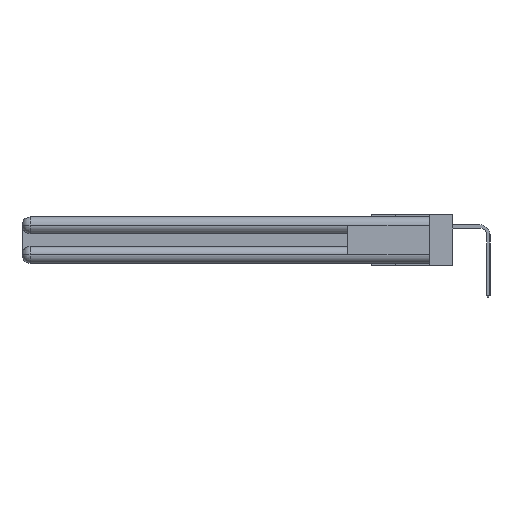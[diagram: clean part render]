
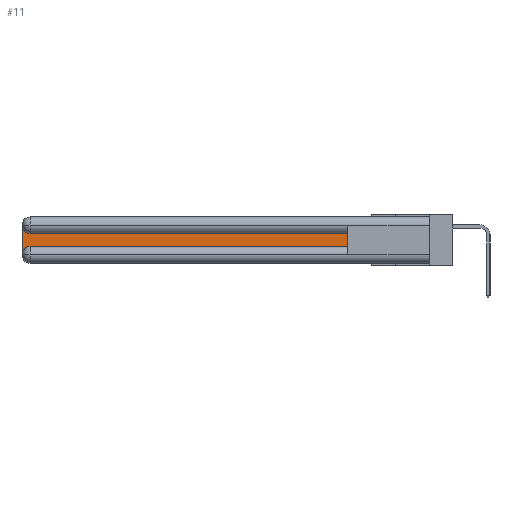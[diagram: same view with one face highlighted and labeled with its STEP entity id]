
A CAD part, left-side view. The second image highlights one B-rep face of the part: STEP entity #11.
In plain terms, the highlighted planar face has unit normal (-1, 0, 0).
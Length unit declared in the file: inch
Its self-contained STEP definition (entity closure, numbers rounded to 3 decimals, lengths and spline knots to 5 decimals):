
#11 = ADVANCED_FACE ( 'NONE', ( #14824 ), #11236, .F. ) ;
#300 = DIRECTION ( 'NONE',  ( 1., 0., 0. ) ) ;
#1218 = DIRECTION ( 'NONE',  ( 1., 0., 0. ) ) ;
#1413 = VECTOR ( 'NONE', #3576, 39.37008 ) ;
#2156 = VECTOR ( 'NONE', #27967, 39.37008 ) ;
#2687 = VECTOR ( 'NONE', #27458, 39.37008 ) ;
#2861 = VERTEX_POINT ( 'NONE', #9665 ) ;
#3286 = ORIENTED_EDGE ( 'NONE', *, *, #26084, .T. ) ;
#3576 = DIRECTION ( 'NONE',  ( 0., 0., 1. ) ) ;
#4928 = LINE ( 'NONE', #28061, #2156 ) ;
#5593 = CARTESIAN_POINT ( 'NONE',  ( 0.075, 0.6, -0.2175 ) ) ;
#7608 = VERTEX_POINT ( 'NONE', #24763 ) ;
#7755 = ORIENTED_EDGE ( 'NONE', *, *, #22667, .T. ) ;
#7760 = DIRECTION ( 'NONE',  ( 0., 0., -1. ) ) ;
#8040 = CARTESIAN_POINT ( 'NONE',  ( 0.075, 2.94, -0.0625 ) ) ;
#8544 = LINE ( 'NONE', #5593, #2687 ) ;
#9607 = VERTEX_POINT ( 'NONE', #18931 ) ;
#9665 = CARTESIAN_POINT ( 'NONE',  ( 0.075, 3., -0.2775 ) ) ;
#9907 = CARTESIAN_POINT ( 'NONE',  ( 0.075, 2.94, -0.2175 ) ) ;
#11236 = PLANE ( 'NONE',  #27590 ) ;
#13456 = CARTESIAN_POINT ( 'NONE',  ( 0.075, 3., -0.1225 ) ) ;
#14821 = ORIENTED_EDGE ( 'NONE', *, *, #15342, .T. ) ;
#14824 = FACE_OUTER_BOUND ( 'NONE', #15076, .T. ) ;
#15076 = EDGE_LOOP ( 'NONE', ( #18240, #7755, #25256, #3286, #21247, #14821 ) ) ;
#15191 = DIRECTION ( 'NONE',  ( 0., 0., -1. ) ) ;
#15342 = EDGE_CURVE ( 'NONE', #9607, #7608, #27272, .T. ) ;
#15680 = DIRECTION ( 'NONE',  ( 0., 0., -1. ) ) ;
#16146 = DIRECTION ( 'NONE',  ( 0., 0., -1. ) ) ;
#16366 = LINE ( 'NONE', #20752, #18421 ) ;
#16428 = EDGE_CURVE ( 'NONE', #7608, #24597, #4928, .T. ) ;
#16748 = CARTESIAN_POINT ( 'NONE',  ( 0.075, 0.6, -0.2175 ) ) ;
#16961 = CARTESIAN_POINT ( 'NONE',  ( 0.075, 3., -0.0625 ) ) ;
#17219 = CARTESIAN_POINT ( 'NONE',  ( 0.075, 2.94, -0.2775 ) ) ;
#18240 = ORIENTED_EDGE ( 'NONE', *, *, #16428, .T. ) ;
#18421 = VECTOR ( 'NONE', #16146, 39.37008 ) ;
#18931 = CARTESIAN_POINT ( 'NONE',  ( 0.075, 0.6, -0.2175 ) ) ;
#19521 = DIRECTION ( 'NONE',  ( 1., 0., 0. ) ) ;
#20752 = CARTESIAN_POINT ( 'NONE',  ( 0.075, 3., -0.2175 ) ) ;
#21247 = ORIENTED_EDGE ( 'NONE', *, *, #24432, .T. ) ;
#22013 = EDGE_CURVE ( 'NONE', #22768, #2861, #16366, .T. ) ;
#22667 = EDGE_CURVE ( 'NONE', #24597, #22768, #28263, .T. ) ;
#22768 = VERTEX_POINT ( 'NONE', #16961 ) ;
#22975 = VERTEX_POINT ( 'NONE', #9907 ) ;
#23909 = CIRCLE ( 'NONE', #27530, 0.06 ) ;
#24432 = EDGE_CURVE ( 'NONE', #22975, #9607, #8544, .T. ) ;
#24597 = VERTEX_POINT ( 'NONE', #26452 ) ;
#24763 = CARTESIAN_POINT ( 'NONE',  ( 0.075, 0.6, -0.1225 ) ) ;
#25256 = ORIENTED_EDGE ( 'NONE', *, *, #22013, .T. ) ;
#26084 = EDGE_CURVE ( 'NONE', #2861, #22975, #23909, .T. ) ;
#26452 = CARTESIAN_POINT ( 'NONE',  ( 0.075, 2.94, -0.1225 ) ) ;
#27097 = AXIS2_PLACEMENT_3D ( 'NONE', #8040, #1218, #7760 ) ;
#27272 = LINE ( 'NONE', #16748, #1413 ) ;
#27458 = DIRECTION ( 'NONE',  ( 0., -1., 0. ) ) ;
#27530 = AXIS2_PLACEMENT_3D ( 'NONE', #17219, #19521, #15191 ) ;
#27590 = AXIS2_PLACEMENT_3D ( 'NONE', #13456, #300, #15680 ) ;
#27967 = DIRECTION ( 'NONE',  ( 0., 1., 0. ) ) ;
#28061 = CARTESIAN_POINT ( 'NONE',  ( 0.075, 0.6, -0.1225 ) ) ;
#28263 = CIRCLE ( 'NONE', #27097, 0.06 ) ;
